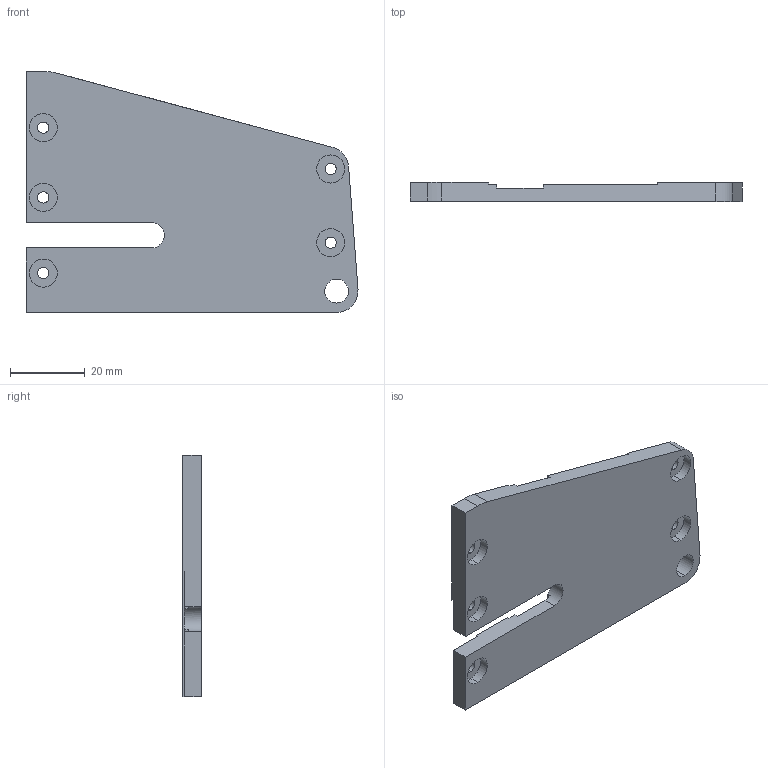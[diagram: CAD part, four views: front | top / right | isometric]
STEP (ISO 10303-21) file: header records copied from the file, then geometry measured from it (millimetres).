
FILE_DESCRIPTION (( 'STEP AP214' ), '1' );
FILE_NAME ('Reinforced_Mag_Well_Left.step', '2015-06-12T17:09:01', ( '' ), ( '' ), 'SwSTEP 2.0', 'SolidWorks 2015', '' );
FILE_SCHEMA (( 'AUTOMOTIVE_DESIGN' ));
Length unit declared in the file: millimetre
Products named in the file (1): Reinforced_Mag_Well_Left
Bounding box: 88.63 x 5 x 64.36 mm (x, y, z)
Volume: 19793.3 mm3; surface area: 11153.5 mm2
Topology: 1 solids, 1 shells, 60 faces, 159 edges, 106 vertices
Faces by surface type: plane 34, cylinder 26
Entity records: 1935 total; most frequent: DIRECTION 335, CARTESIAN_POINT 326, ORIENTED_EDGE 318, EDGE_CURVE 159, AXIS2_PLACEMENT_3D 115, VERTEX_POINT 106, VECTOR 105, LINE 105
